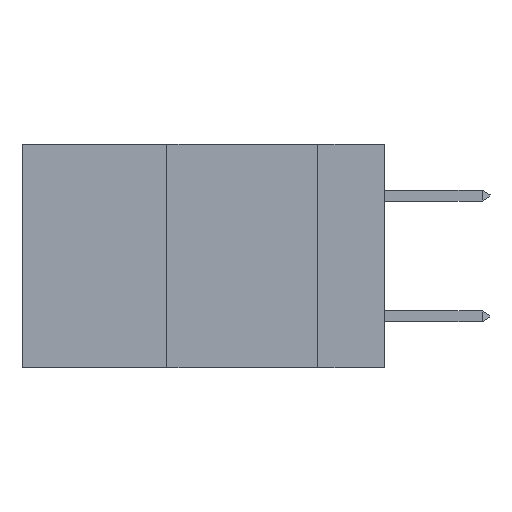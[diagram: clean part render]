
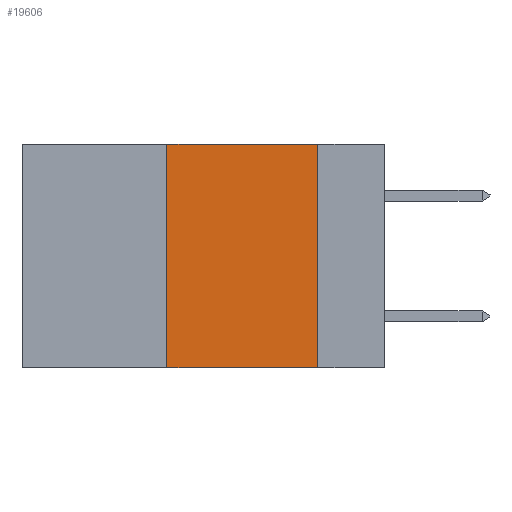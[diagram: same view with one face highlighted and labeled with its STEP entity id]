
A CAD part, left-side view. The second image highlights one B-rep face of the part: STEP entity #19606.
In plain terms, the highlighted planar face has unit normal (-1, 0, 0).
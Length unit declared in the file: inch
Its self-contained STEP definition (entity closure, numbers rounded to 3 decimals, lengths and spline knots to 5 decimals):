
#119 = ORIENTED_EDGE ( 'NONE', *, *, #18512, .F. ) ;
#1116 = EDGE_CURVE ( 'NONE', #13958, #21160, #20648, .T. ) ;
#1295 = DIRECTION ( 'NONE',  ( 0., 0., -1. ) ) ;
#2209 = LINE ( 'NONE', #2613, #16487 ) ;
#2327 = CARTESIAN_POINT ( 'NONE',  ( 0., 0.11, 0. ) ) ;
#2374 = LINE ( 'NONE', #6823, #12994 ) ;
#2613 = CARTESIAN_POINT ( 'NONE',  ( 0., 0.36, 0. ) ) ;
#5298 = EDGE_CURVE ( 'NONE', #16846, #7056, #2374, .T. ) ;
#5307 = FACE_OUTER_BOUND ( 'NONE', #19037, .T. ) ;
#6014 = PLANE ( 'NONE',  #9611 ) ;
#6373 = EDGE_CURVE ( 'NONE', #21160, #7056, #19990, .T. ) ;
#6823 = CARTESIAN_POINT ( 'NONE',  ( 0., 0.6, -0.37 ) ) ;
#7056 = VERTEX_POINT ( 'NONE', #10656 ) ;
#8060 = CARTESIAN_POINT ( 'NONE',  ( 0., 0.6, 0. ) ) ;
#8219 = CARTESIAN_POINT ( 'NONE',  ( 0., 0.11, 0. ) ) ;
#9327 = CARTESIAN_POINT ( 'NONE',  ( 0., 0.6, 0. ) ) ;
#9611 = AXIS2_PLACEMENT_3D ( 'NONE', #9327, #14441, #1295 ) ;
#9921 = DIRECTION ( 'NONE',  ( 0., -1., 0. ) ) ;
#10488 = ORIENTED_EDGE ( 'NONE', *, *, #5298, .T. ) ;
#10656 = CARTESIAN_POINT ( 'NONE',  ( 0., 0.11, -0.37 ) ) ;
#10996 = DIRECTION ( 'NONE',  ( 0., 0., 1. ) ) ;
#12584 = ORIENTED_EDGE ( 'NONE', *, *, #6373, .F. ) ;
#12994 = VECTOR ( 'NONE', #14966, 39.37008 ) ;
#13233 = VECTOR ( 'NONE', #17500, 39.37008 ) ;
#13958 = VERTEX_POINT ( 'NONE', #19789 ) ;
#14441 = DIRECTION ( 'NONE',  ( 1., 0., 0. ) ) ;
#14966 = DIRECTION ( 'NONE',  ( 0., -1., 0. ) ) ;
#15186 = VECTOR ( 'NONE', #9921, 39.37008 ) ;
#15552 = CARTESIAN_POINT ( 'NONE',  ( 0., 0.36, -0.37 ) ) ;
#16487 = VECTOR ( 'NONE', #10996, 39.37008 ) ;
#16846 = VERTEX_POINT ( 'NONE', #15552 ) ;
#17500 = DIRECTION ( 'NONE',  ( 0., 0., -1. ) ) ;
#18512 = EDGE_CURVE ( 'NONE', #16846, #13958, #2209, .T. ) ;
#19037 = EDGE_LOOP ( 'NONE', ( #12584, #20375, #119, #10488 ) ) ;
#19606 = ADVANCED_FACE ( 'NONE', ( #5307 ), #6014, .F. ) ;
#19789 = CARTESIAN_POINT ( 'NONE',  ( 0., 0.36, 0. ) ) ;
#19990 = LINE ( 'NONE', #2327, #13233 ) ;
#20375 = ORIENTED_EDGE ( 'NONE', *, *, #1116, .F. ) ;
#20648 = LINE ( 'NONE', #8060, #15186 ) ;
#21160 = VERTEX_POINT ( 'NONE', #8219 ) ;
